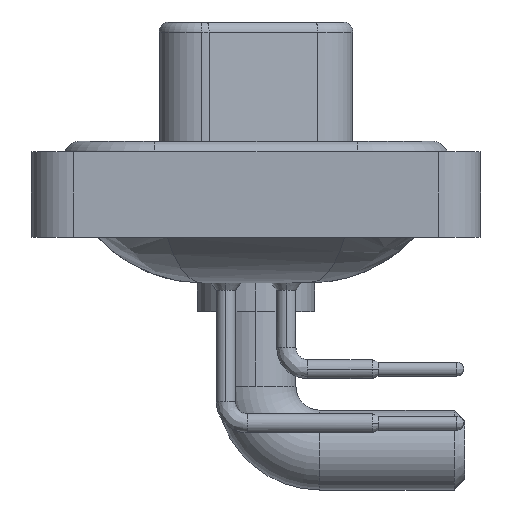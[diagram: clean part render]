
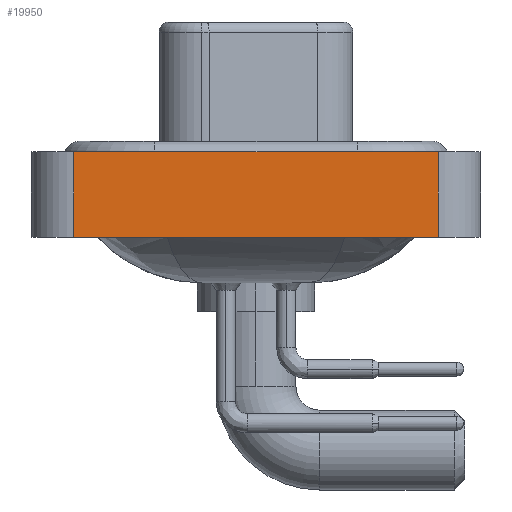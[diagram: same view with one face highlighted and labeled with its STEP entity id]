
A CAD part, left-side view. The second image highlights one B-rep face of the part: STEP entity #19950.
In plain terms, the highlighted planar face has unit normal (-1, 0, 0).
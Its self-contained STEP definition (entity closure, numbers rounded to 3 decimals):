
#140 = CARTESIAN_POINT ( 'NONE',  ( -7.35, -8.55, -3.6 ) ) ;
#554 = EDGE_CURVE ( 'NONE', #25155, #14025, #12497, .T. ) ;
#611 = CARTESIAN_POINT ( 'NONE',  ( -7.35, 8.55, -3.6 ) ) ;
#793 = EDGE_CURVE ( 'NONE', #25155, #7524, #14530, .T. ) ;
#839 = EDGE_LOOP ( 'NONE', ( #23574, #29513, #21739, #21499 ) ) ;
#2799 = EDGE_CURVE ( 'NONE', #14025, #8263, #5954, .T. ) ;
#3712 = DIRECTION ( 'NONE',  ( 0., 0., 1. ) ) ;
#3909 = CARTESIAN_POINT ( 'NONE',  ( -7.35, -8.55, 0.4 ) ) ;
#4923 = DIRECTION ( 'NONE',  ( 0., 0., 1. ) ) ;
#5954 = LINE ( 'NONE', #15072, #11587 ) ;
#7524 = VERTEX_POINT ( 'NONE', #11194 ) ;
#8147 = CARTESIAN_POINT ( 'NONE',  ( -7.35, -8.55, 0.4 ) ) ;
#8263 = VERTEX_POINT ( 'NONE', #3909 ) ;
#9536 = EDGE_CURVE ( 'NONE', #7524, #8263, #16971, .T. ) ;
#11194 = CARTESIAN_POINT ( 'NONE',  ( -7.35, 8.55, 0.4 ) ) ;
#11587 = VECTOR ( 'NONE', #3712, 1000. ) ;
#12497 = LINE ( 'NONE', #21939, #22490 ) ;
#13506 = VECTOR ( 'NONE', #28360, 1000. ) ;
#14025 = VERTEX_POINT ( 'NONE', #14225 ) ;
#14225 = CARTESIAN_POINT ( 'NONE',  ( -7.35, -8.55, -3.6 ) ) ;
#14530 = LINE ( 'NONE', #611, #23915 ) ;
#15072 = CARTESIAN_POINT ( 'NONE',  ( -7.35, -8.55, -3.6 ) ) ;
#16773 = DIRECTION ( 'NONE',  ( 0., 0., 1. ) ) ;
#16971 = LINE ( 'NONE', #8147, #13506 ) ;
#18561 = PLANE ( 'NONE',  #24211 ) ;
#19678 = CARTESIAN_POINT ( 'NONE',  ( -7.35, 8.55, -3.6 ) ) ;
#19950 = ADVANCED_FACE ( 'NONE', ( #20673 ), #18561, .T. ) ;
#20673 = FACE_OUTER_BOUND ( 'NONE', #839, .T. ) ;
#21499 = ORIENTED_EDGE ( 'NONE', *, *, #554, .T. ) ;
#21739 = ORIENTED_EDGE ( 'NONE', *, *, #793, .F. ) ;
#21939 = CARTESIAN_POINT ( 'NONE',  ( -7.35, -8.55, -3.6 ) ) ;
#22490 = VECTOR ( 'NONE', #24026, 1000. ) ;
#23574 = ORIENTED_EDGE ( 'NONE', *, *, #2799, .T. ) ;
#23915 = VECTOR ( 'NONE', #16773, 1000. ) ;
#24026 = DIRECTION ( 'NONE',  ( 0., -1., 0. ) ) ;
#24211 = AXIS2_PLACEMENT_3D ( 'NONE', #140, #27697, #4923 ) ;
#25155 = VERTEX_POINT ( 'NONE', #19678 ) ;
#27697 = DIRECTION ( 'NONE',  ( -1., 0., 0. ) ) ;
#28360 = DIRECTION ( 'NONE',  ( 0., -1., 0. ) ) ;
#29513 = ORIENTED_EDGE ( 'NONE', *, *, #9536, .F. ) ;
